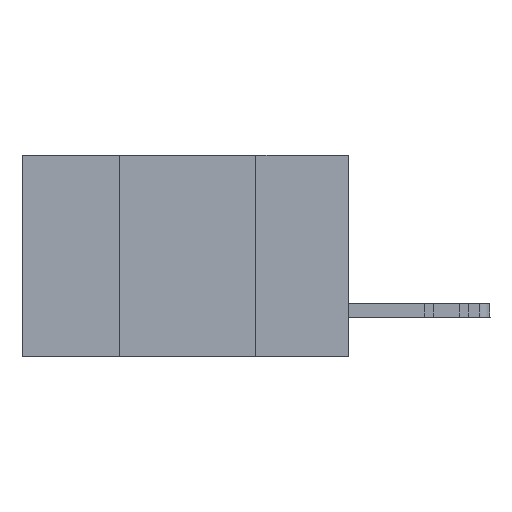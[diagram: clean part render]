
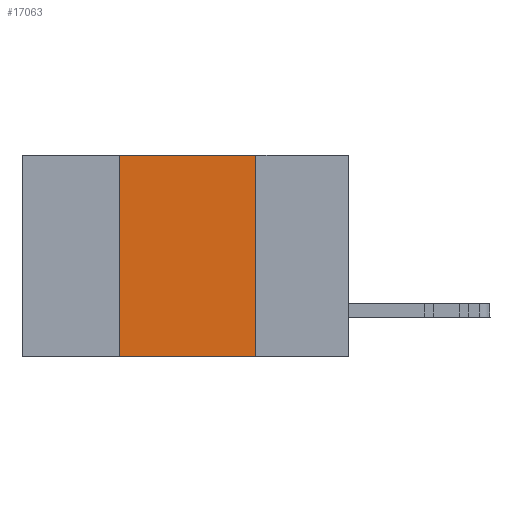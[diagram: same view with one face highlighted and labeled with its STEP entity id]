
A CAD part, left-side view. The second image highlights one B-rep face of the part: STEP entity #17063.
In plain terms, the highlighted planar face has unit normal (-1, 0, 0).
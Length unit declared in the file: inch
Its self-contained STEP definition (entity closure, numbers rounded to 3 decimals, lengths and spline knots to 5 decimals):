
#1972 = DIRECTION ( 'NONE',  ( 0., -1., 0. ) ) ;
#2334 = VECTOR ( 'NONE', #14010, 39.37008 ) ;
#3006 = DIRECTION ( 'NONE',  ( 0., 0., -1. ) ) ;
#4402 = CARTESIAN_POINT ( 'NONE',  ( 0., 0.6, 0. ) ) ;
#5532 = VECTOR ( 'NONE', #7162, 39.37008 ) ;
#6005 = ORIENTED_EDGE ( 'NONE', *, *, #16124, .F. ) ;
#6667 = VERTEX_POINT ( 'NONE', #15018 ) ;
#6727 = LINE ( 'NONE', #4402, #5532 ) ;
#6733 = CARTESIAN_POINT ( 'NONE',  ( 0., 0.42, 0. ) ) ;
#7162 = DIRECTION ( 'NONE',  ( 0., -1., 0. ) ) ;
#7388 = FACE_OUTER_BOUND ( 'NONE', #8746, .T. ) ;
#7492 = AXIS2_PLACEMENT_3D ( 'NONE', #20518, #14083, #3006 ) ;
#8746 = EDGE_LOOP ( 'NONE', ( #24995, #25762, #6005, #28709 ) ) ;
#8760 = CARTESIAN_POINT ( 'NONE',  ( 0., 0.17, 0. ) ) ;
#8826 = DIRECTION ( 'NONE',  ( 0., 0., -1. ) ) ;
#12407 = CARTESIAN_POINT ( 'NONE',  ( 0., 0.42, -0.37 ) ) ;
#14010 = DIRECTION ( 'NONE',  ( 0., 0., 1. ) ) ;
#14083 = DIRECTION ( 'NONE',  ( 1., 0., 0. ) ) ;
#14790 = EDGE_CURVE ( 'NONE', #6667, #18269, #6727, .T. ) ;
#15018 = CARTESIAN_POINT ( 'NONE',  ( 0., 0.42, 0. ) ) ;
#15876 = VECTOR ( 'NONE', #8826, 39.37008 ) ;
#16124 = EDGE_CURVE ( 'NONE', #19771, #6667, #27167, .T. ) ;
#16145 = PLANE ( 'NONE',  #7492 ) ;
#17063 = ADVANCED_FACE ( 'NONE', ( #7388 ), #16145, .F. ) ;
#17512 = EDGE_CURVE ( 'NONE', #18269, #27814, #28682, .T. ) ;
#18269 = VERTEX_POINT ( 'NONE', #8760 ) ;
#18727 = VECTOR ( 'NONE', #1972, 39.37008 ) ;
#19182 = EDGE_CURVE ( 'NONE', #19771, #27814, #19353, .T. ) ;
#19353 = LINE ( 'NONE', #26061, #18727 ) ;
#19771 = VERTEX_POINT ( 'NONE', #12407 ) ;
#20518 = CARTESIAN_POINT ( 'NONE',  ( 0., 0.6, 0. ) ) ;
#21794 = CARTESIAN_POINT ( 'NONE',  ( 0., 0.17, -0.37 ) ) ;
#24995 = ORIENTED_EDGE ( 'NONE', *, *, #17512, .F. ) ;
#25762 = ORIENTED_EDGE ( 'NONE', *, *, #14790, .F. ) ;
#26061 = CARTESIAN_POINT ( 'NONE',  ( 0., 0.6, -0.37 ) ) ;
#27167 = LINE ( 'NONE', #6733, #2334 ) ;
#27814 = VERTEX_POINT ( 'NONE', #21794 ) ;
#28682 = LINE ( 'NONE', #28821, #15876 ) ;
#28709 = ORIENTED_EDGE ( 'NONE', *, *, #19182, .T. ) ;
#28821 = CARTESIAN_POINT ( 'NONE',  ( 0., 0.17, 0. ) ) ;
